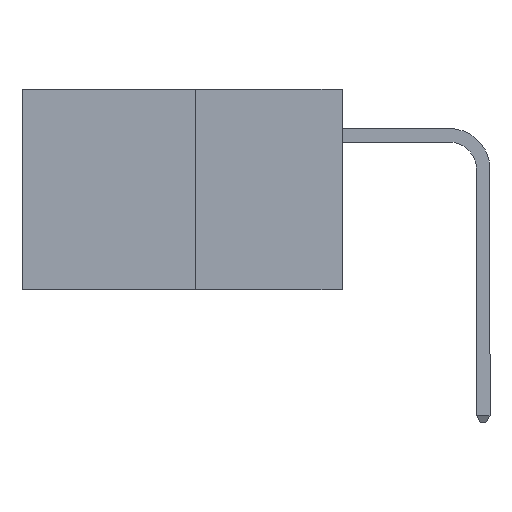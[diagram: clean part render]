
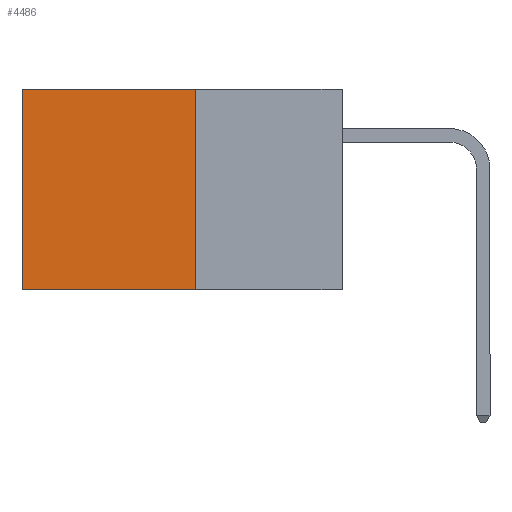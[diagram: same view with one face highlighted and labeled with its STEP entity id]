
A CAD part, left-side view. The second image highlights one B-rep face of the part: STEP entity #4486.
In plain terms, the highlighted planar face has unit normal (-1, 0, 0).
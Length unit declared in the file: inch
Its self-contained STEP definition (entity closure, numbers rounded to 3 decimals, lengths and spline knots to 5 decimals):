
#92 = VECTOR ( 'NONE', #2345, 39.37008 ) ;
#249 = VECTOR ( 'NONE', #2224, 39.37008 ) ;
#450 = LINE ( 'NONE', #5490, #7891 ) ;
#496 = CARTESIAN_POINT ( 'NONE',  ( 0.277, 0.59, 0. ) ) ;
#628 = CARTESIAN_POINT ( 'NONE',  ( 0.277, 0.59, -0.37 ) ) ;
#1064 = CARTESIAN_POINT ( 'NONE',  ( 0.277, 0.59, -0.37 ) ) ;
#1404 = ORIENTED_EDGE ( 'NONE', *, *, #5261, .T. ) ;
#1542 = EDGE_LOOP ( 'NONE', ( #6490, #3569, #2436, #1404 ) ) ;
#1673 = CARTESIAN_POINT ( 'NONE',  ( 0.277, 0.27, -0.37 ) ) ;
#2224 = DIRECTION ( 'NONE',  ( 0., 1., 0. ) ) ;
#2269 = DIRECTION ( 'NONE',  ( 0., 0., -1. ) ) ;
#2345 = DIRECTION ( 'NONE',  ( 0., 0., -1. ) ) ;
#2436 = ORIENTED_EDGE ( 'NONE', *, *, #2460, .F. ) ;
#2455 = DIRECTION ( 'NONE',  ( 0., 1., 0. ) ) ;
#2460 = EDGE_CURVE ( 'NONE', #5920, #4672, #450, .T. ) ;
#2603 = CARTESIAN_POINT ( 'NONE',  ( 0.277, 0.27, -0.37 ) ) ;
#3108 = EDGE_CURVE ( 'NONE', #4655, #8674, #7538, .T. ) ;
#3563 = VECTOR ( 'NONE', #2455, 39.37008 ) ;
#3569 = ORIENTED_EDGE ( 'NONE', *, *, #5945, .F. ) ;
#3734 = PLANE ( 'NONE',  #4496 ) ;
#3975 = DIRECTION ( 'NONE',  ( 0., 0., -1. ) ) ;
#4486 = ADVANCED_FACE ( 'NONE', ( #7040 ), #3734, .F. ) ;
#4496 = AXIS2_PLACEMENT_3D ( 'NONE', #2603, #8380, #3975 ) ;
#4644 = CARTESIAN_POINT ( 'NONE',  ( 0.277, 0.27, -0.37 ) ) ;
#4655 = VERTEX_POINT ( 'NONE', #496 ) ;
#4672 = VERTEX_POINT ( 'NONE', #1673 ) ;
#5261 = EDGE_CURVE ( 'NONE', #5920, #4655, #7689, .T. ) ;
#5490 = CARTESIAN_POINT ( 'NONE',  ( 0.277, 0.27, -0.37 ) ) ;
#5906 = CARTESIAN_POINT ( 'NONE',  ( 0.277, 0.27, 0. ) ) ;
#5920 = VERTEX_POINT ( 'NONE', #5906 ) ;
#5926 = CARTESIAN_POINT ( 'NONE',  ( 0.277, 0.27, 0. ) ) ;
#5945 = EDGE_CURVE ( 'NONE', #4672, #8674, #7557, .T. ) ;
#6490 = ORIENTED_EDGE ( 'NONE', *, *, #3108, .T. ) ;
#7040 = FACE_OUTER_BOUND ( 'NONE', #1542, .T. ) ;
#7538 = LINE ( 'NONE', #628, #92 ) ;
#7557 = LINE ( 'NONE', #4644, #3563 ) ;
#7689 = LINE ( 'NONE', #5926, #249 ) ;
#7891 = VECTOR ( 'NONE', #2269, 39.37008 ) ;
#8380 = DIRECTION ( 'NONE',  ( 1., 0., 0. ) ) ;
#8674 = VERTEX_POINT ( 'NONE', #1064 ) ;
